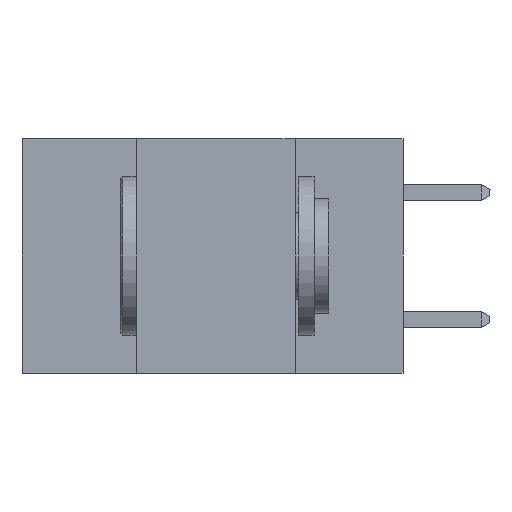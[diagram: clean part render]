
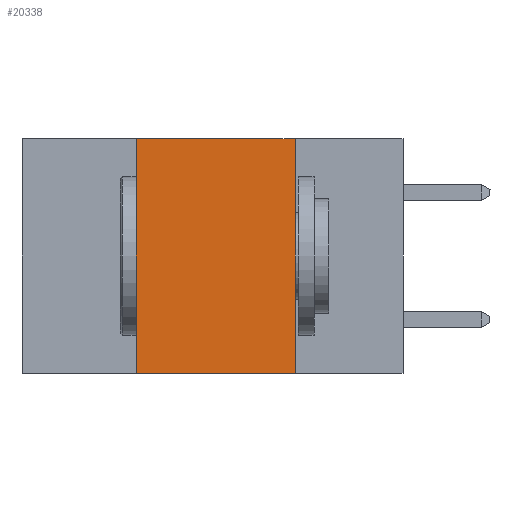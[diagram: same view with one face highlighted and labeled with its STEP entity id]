
A CAD part, left-side view. The second image highlights one B-rep face of the part: STEP entity #20338.
In plain terms, the highlighted planar face has unit normal (-1, 0, 0).
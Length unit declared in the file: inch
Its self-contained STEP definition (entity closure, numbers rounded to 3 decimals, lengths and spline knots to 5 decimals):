
#1303 = EDGE_CURVE ( 'NONE', #7373, #19132, #5946, .T. ) ;
#1734 = CARTESIAN_POINT ( 'NONE',  ( 0., 0.17, -0.37 ) ) ;
#2355 = EDGE_LOOP ( 'NONE', ( #3630, #17984, #22854, #14996 ) ) ;
#2681 = CARTESIAN_POINT ( 'NONE',  ( 0., 0.42, 0. ) ) ;
#2908 = EDGE_CURVE ( 'NONE', #7105, #20778, #9689, .T. ) ;
#3296 = FACE_OUTER_BOUND ( 'NONE', #2355, .T. ) ;
#3630 = ORIENTED_EDGE ( 'NONE', *, *, #2908, .F. ) ;
#4471 = VECTOR ( 'NONE', #22084, 39.37008 ) ;
#4525 = CARTESIAN_POINT ( 'NONE',  ( 0., 0.6, 0. ) ) ;
#5946 = LINE ( 'NONE', #17637, #22132 ) ;
#6207 = EDGE_CURVE ( 'NONE', #7373, #20778, #7696, .T. ) ;
#6473 = VECTOR ( 'NONE', #9652, 39.37008 ) ;
#6494 = PLANE ( 'NONE',  #13604 ) ;
#7105 = VERTEX_POINT ( 'NONE', #12979 ) ;
#7373 = VERTEX_POINT ( 'NONE', #16144 ) ;
#7696 = LINE ( 'NONE', #25211, #6473 ) ;
#7958 = EDGE_CURVE ( 'NONE', #19132, #7105, #21314, .T. ) ;
#9652 = DIRECTION ( 'NONE',  ( 0., -1., 0. ) ) ;
#9689 = LINE ( 'NONE', #22553, #4471 ) ;
#10438 = DIRECTION ( 'NONE',  ( 0., 0., -1. ) ) ;
#12979 = CARTESIAN_POINT ( 'NONE',  ( 0., 0.17, 0. ) ) ;
#13604 = AXIS2_PLACEMENT_3D ( 'NONE', #4525, #22102, #10438 ) ;
#14996 = ORIENTED_EDGE ( 'NONE', *, *, #6207, .T. ) ;
#16144 = CARTESIAN_POINT ( 'NONE',  ( 0., 0.42, -0.37 ) ) ;
#16163 = VECTOR ( 'NONE', #21882, 39.37008 ) ;
#17637 = CARTESIAN_POINT ( 'NONE',  ( 0., 0.42, 0. ) ) ;
#17697 = DIRECTION ( 'NONE',  ( 0., 0., 1. ) ) ;
#17965 = CARTESIAN_POINT ( 'NONE',  ( 0., 0.6, 0. ) ) ;
#17984 = ORIENTED_EDGE ( 'NONE', *, *, #7958, .F. ) ;
#19132 = VERTEX_POINT ( 'NONE', #2681 ) ;
#20338 = ADVANCED_FACE ( 'NONE', ( #3296 ), #6494, .F. ) ;
#20778 = VERTEX_POINT ( 'NONE', #1734 ) ;
#21314 = LINE ( 'NONE', #17965, #16163 ) ;
#21882 = DIRECTION ( 'NONE',  ( 0., -1., 0. ) ) ;
#22084 = DIRECTION ( 'NONE',  ( 0., 0., -1. ) ) ;
#22102 = DIRECTION ( 'NONE',  ( 1., 0., 0. ) ) ;
#22132 = VECTOR ( 'NONE', #17697, 39.37008 ) ;
#22553 = CARTESIAN_POINT ( 'NONE',  ( 0., 0.17, 0. ) ) ;
#22854 = ORIENTED_EDGE ( 'NONE', *, *, #1303, .F. ) ;
#25211 = CARTESIAN_POINT ( 'NONE',  ( 0., 0.6, -0.37 ) ) ;
